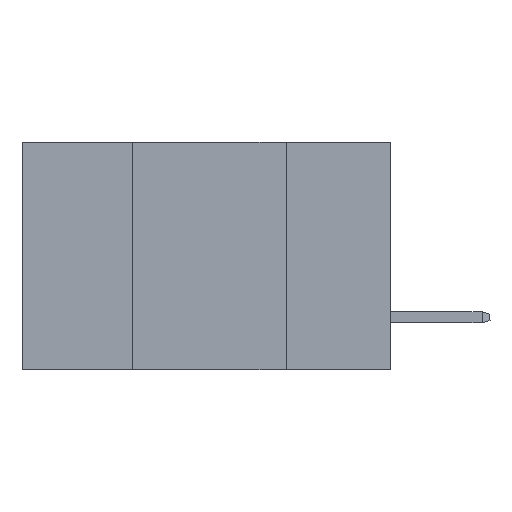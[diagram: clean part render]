
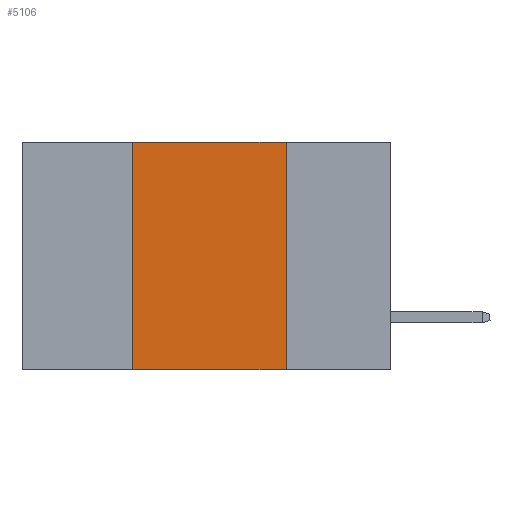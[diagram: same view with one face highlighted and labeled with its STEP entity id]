
A CAD part, left-side view. The second image highlights one B-rep face of the part: STEP entity #5106.
In plain terms, the highlighted planar face has unit normal (-1, 0, 0).
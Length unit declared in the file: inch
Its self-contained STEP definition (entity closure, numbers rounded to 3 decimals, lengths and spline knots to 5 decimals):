
#68 = VERTEX_POINT ( 'NONE', #9075 ) ;
#962 = VECTOR ( 'NONE', #11698, 39.37008 ) ;
#1304 = CARTESIAN_POINT ( 'NONE',  ( 0., 0.6, 0. ) ) ;
#1627 = DIRECTION ( 'NONE',  ( 0., -1., 0. ) ) ;
#1962 = EDGE_CURVE ( 'NONE', #5687, #4267, #5129, .T. ) ;
#2119 = CARTESIAN_POINT ( 'NONE',  ( 0., 0.42, 0. ) ) ;
#2176 = VERTEX_POINT ( 'NONE', #6341 ) ;
#2267 = DIRECTION ( 'NONE',  ( 1., 0., 0. ) ) ;
#4160 = DIRECTION ( 'NONE',  ( 0., 0., 1. ) ) ;
#4267 = VERTEX_POINT ( 'NONE', #9894 ) ;
#4426 = LINE ( 'NONE', #6096, #11157 ) ;
#4853 = LINE ( 'NONE', #8041, #7111 ) ;
#4874 = EDGE_CURVE ( 'NONE', #2176, #68, #6101, .T. ) ;
#5106 = ADVANCED_FACE ( 'NONE', ( #6245 ), #8020, .F. ) ;
#5129 = LINE ( 'NONE', #8973, #7384 ) ;
#5687 = VERTEX_POINT ( 'NONE', #2119 ) ;
#5759 = EDGE_CURVE ( 'NONE', #2176, #5687, #4426, .T. ) ;
#6096 = CARTESIAN_POINT ( 'NONE',  ( 0., 0.42, 0. ) ) ;
#6101 = LINE ( 'NONE', #9789, #962 ) ;
#6245 = FACE_OUTER_BOUND ( 'NONE', #11825, .T. ) ;
#6341 = CARTESIAN_POINT ( 'NONE',  ( 0., 0.42, -0.37 ) ) ;
#6408 = EDGE_CURVE ( 'NONE', #4267, #68, #4853, .T. ) ;
#7111 = VECTOR ( 'NONE', #10933, 39.37008 ) ;
#7384 = VECTOR ( 'NONE', #1627, 39.37008 ) ;
#8020 = PLANE ( 'NONE',  #9282 ) ;
#8041 = CARTESIAN_POINT ( 'NONE',  ( 0., 0.17, 0. ) ) ;
#8973 = CARTESIAN_POINT ( 'NONE',  ( 0., 0.6, 0. ) ) ;
#8991 = DIRECTION ( 'NONE',  ( 0., 0., -1. ) ) ;
#9075 = CARTESIAN_POINT ( 'NONE',  ( 0., 0.17, -0.37 ) ) ;
#9237 = ORIENTED_EDGE ( 'NONE', *, *, #1962, .F. ) ;
#9282 = AXIS2_PLACEMENT_3D ( 'NONE', #1304, #2267, #8991 ) ;
#9538 = ORIENTED_EDGE ( 'NONE', *, *, #5759, .F. ) ;
#9789 = CARTESIAN_POINT ( 'NONE',  ( 0., 0.6, -0.37 ) ) ;
#9894 = CARTESIAN_POINT ( 'NONE',  ( 0., 0.17, 0. ) ) ;
#10933 = DIRECTION ( 'NONE',  ( 0., 0., -1. ) ) ;
#11157 = VECTOR ( 'NONE', #4160, 39.37008 ) ;
#11477 = ORIENTED_EDGE ( 'NONE', *, *, #6408, .F. ) ;
#11698 = DIRECTION ( 'NONE',  ( 0., -1., 0. ) ) ;
#11825 = EDGE_LOOP ( 'NONE', ( #11477, #9237, #9538, #12365 ) ) ;
#12365 = ORIENTED_EDGE ( 'NONE', *, *, #4874, .T. ) ;
